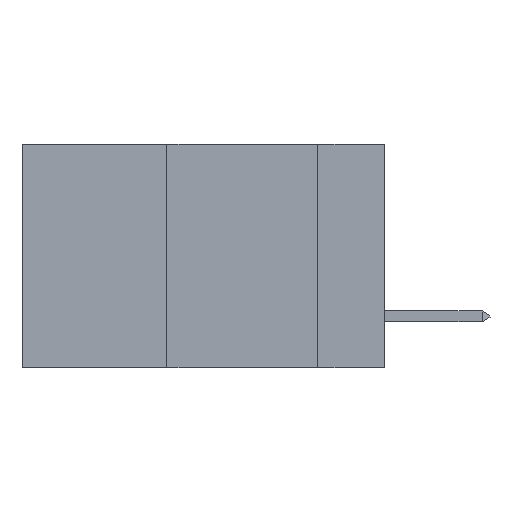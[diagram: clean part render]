
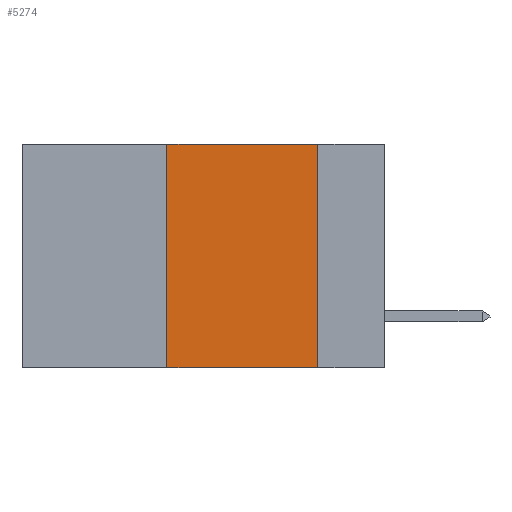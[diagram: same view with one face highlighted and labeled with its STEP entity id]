
A CAD part, left-side view. The second image highlights one B-rep face of the part: STEP entity #5274.
In plain terms, the highlighted planar face has unit normal (-1, 0, 0).
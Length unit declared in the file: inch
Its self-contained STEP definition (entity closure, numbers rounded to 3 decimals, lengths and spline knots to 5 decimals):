
#907 = EDGE_CURVE ( 'NONE', #14998, #25941, #1861, .T. ) ;
#1271 = VERTEX_POINT ( 'NONE', #17605 ) ;
#1272 = VECTOR ( 'NONE', #5899, 39.37008 ) ;
#1718 = DIRECTION ( 'NONE',  ( 0., 0., -1. ) ) ;
#1861 = LINE ( 'NONE', #16336, #19218 ) ;
#2166 = ORIENTED_EDGE ( 'NONE', *, *, #907, .F. ) ;
#5274 = ADVANCED_FACE ( 'NONE', ( #16810 ), #26553, .F. ) ;
#5899 = DIRECTION ( 'NONE',  ( 0., 0., -1. ) ) ;
#7347 = VECTOR ( 'NONE', #29358, 39.37008 ) ;
#7348 = DIRECTION ( 'NONE',  ( 0., 0., 1. ) ) ;
#11314 = CARTESIAN_POINT ( 'NONE',  ( 0., 0.6, -0.37 ) ) ;
#13059 = CARTESIAN_POINT ( 'NONE',  ( 0., 0.6, 0. ) ) ;
#14465 = EDGE_CURVE ( 'NONE', #14998, #1271, #18644, .T. ) ;
#14926 = EDGE_CURVE ( 'NONE', #25941, #19570, #23902, .T. ) ;
#14998 = VERTEX_POINT ( 'NONE', #29030 ) ;
#15264 = ORIENTED_EDGE ( 'NONE', *, *, #14465, .T. ) ;
#15309 = DIRECTION ( 'NONE',  ( 1., 0., 0. ) ) ;
#16336 = CARTESIAN_POINT ( 'NONE',  ( 0., 0.36, 0. ) ) ;
#16810 = FACE_OUTER_BOUND ( 'NONE', #17112, .T. ) ;
#17112 = EDGE_LOOP ( 'NONE', ( #22158, #22206, #2166, #15264 ) ) ;
#17159 = CARTESIAN_POINT ( 'NONE',  ( 0., 0.11, 0. ) ) ;
#17209 = VECTOR ( 'NONE', #28740, 39.37008 ) ;
#17507 = CARTESIAN_POINT ( 'NONE',  ( 0., 0.6, 0. ) ) ;
#17605 = CARTESIAN_POINT ( 'NONE',  ( 0., 0.11, -0.37 ) ) ;
#18644 = LINE ( 'NONE', #11314, #7347 ) ;
#19218 = VECTOR ( 'NONE', #7348, 39.37008 ) ;
#19570 = VERTEX_POINT ( 'NONE', #22207 ) ;
#20070 = EDGE_CURVE ( 'NONE', #19570, #1271, #20082, .T. ) ;
#20082 = LINE ( 'NONE', #17159, #1272 ) ;
#21146 = AXIS2_PLACEMENT_3D ( 'NONE', #13059, #15309, #1718 ) ;
#22158 = ORIENTED_EDGE ( 'NONE', *, *, #20070, .F. ) ;
#22206 = ORIENTED_EDGE ( 'NONE', *, *, #14926, .F. ) ;
#22207 = CARTESIAN_POINT ( 'NONE',  ( 0., 0.11, 0. ) ) ;
#23902 = LINE ( 'NONE', #17507, #17209 ) ;
#24826 = CARTESIAN_POINT ( 'NONE',  ( 0., 0.36, 0. ) ) ;
#25941 = VERTEX_POINT ( 'NONE', #24826 ) ;
#26553 = PLANE ( 'NONE',  #21146 ) ;
#28740 = DIRECTION ( 'NONE',  ( 0., -1., 0. ) ) ;
#29030 = CARTESIAN_POINT ( 'NONE',  ( 0., 0.36, -0.37 ) ) ;
#29358 = DIRECTION ( 'NONE',  ( 0., -1., 0. ) ) ;
